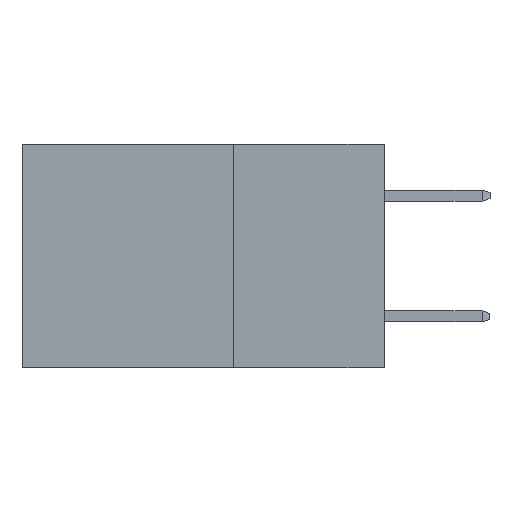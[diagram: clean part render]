
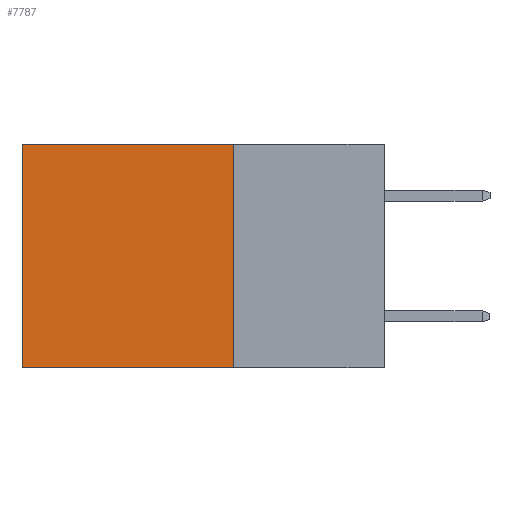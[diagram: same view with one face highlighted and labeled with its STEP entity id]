
A CAD part, left-side view. The second image highlights one B-rep face of the part: STEP entity #7787.
In plain terms, the highlighted planar face has unit normal (-1, 0, 0).
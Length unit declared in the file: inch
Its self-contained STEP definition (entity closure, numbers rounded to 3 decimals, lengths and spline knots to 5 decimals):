
#214 = AXIS2_PLACEMENT_3D ( 'NONE', #4296, #17060, #8611 ) ;
#1659 = LINE ( 'NONE', #11993, #5017 ) ;
#1686 = VERTEX_POINT ( 'NONE', #16379 ) ;
#1791 = CARTESIAN_POINT ( 'NONE',  ( 0.298, 0.6, 0. ) ) ;
#2980 = CARTESIAN_POINT ( 'NONE',  ( 0.298, 0.25, 0. ) ) ;
#3891 = VERTEX_POINT ( 'NONE', #1791 ) ;
#4040 = EDGE_CURVE ( 'NONE', #16604, #3891, #4659, .T. ) ;
#4296 = CARTESIAN_POINT ( 'NONE',  ( 0.298, 0.25, 0. ) ) ;
#4659 = LINE ( 'NONE', #2980, #15600 ) ;
#4667 = DIRECTION ( 'NONE',  ( 0., 1., 0. ) ) ;
#5017 = VECTOR ( 'NONE', #12271, 39.37008 ) ;
#5108 = LINE ( 'NONE', #11768, #16018 ) ;
#6011 = DIRECTION ( 'NONE',  ( 0., 1., 0. ) ) ;
#6279 = EDGE_CURVE ( 'NONE', #16604, #1686, #1659, .T. ) ;
#7108 = CARTESIAN_POINT ( 'NONE',  ( 0.298, 0.6, -0.37 ) ) ;
#7216 = FACE_OUTER_BOUND ( 'NONE', #8972, .T. ) ;
#7787 = ADVANCED_FACE ( 'NONE', ( #7216 ), #8556, .F. ) ;
#8025 = VECTOR ( 'NONE', #14995, 39.37008 ) ;
#8301 = ORIENTED_EDGE ( 'NONE', *, *, #18335, .F. ) ;
#8480 = LINE ( 'NONE', #16353, #8025 ) ;
#8556 = PLANE ( 'NONE',  #214 ) ;
#8611 = DIRECTION ( 'NONE',  ( 0., 0., -1. ) ) ;
#8972 = EDGE_LOOP ( 'NONE', ( #10020, #8301, #13234, #10980 ) ) ;
#9854 = VERTEX_POINT ( 'NONE', #7108 ) ;
#10020 = ORIENTED_EDGE ( 'NONE', *, *, #11534, .T. ) ;
#10980 = ORIENTED_EDGE ( 'NONE', *, *, #4040, .T. ) ;
#11534 = EDGE_CURVE ( 'NONE', #3891, #9854, #8480, .T. ) ;
#11768 = CARTESIAN_POINT ( 'NONE',  ( 0.298, 0.25, -0.37 ) ) ;
#11993 = CARTESIAN_POINT ( 'NONE',  ( 0.298, 0.25, 0. ) ) ;
#12271 = DIRECTION ( 'NONE',  ( 0., 0., -1. ) ) ;
#13234 = ORIENTED_EDGE ( 'NONE', *, *, #6279, .F. ) ;
#14995 = DIRECTION ( 'NONE',  ( 0., 0., -1. ) ) ;
#15600 = VECTOR ( 'NONE', #4667, 39.37008 ) ;
#16018 = VECTOR ( 'NONE', #6011, 39.37008 ) ;
#16353 = CARTESIAN_POINT ( 'NONE',  ( 0.298, 0.6, 0. ) ) ;
#16379 = CARTESIAN_POINT ( 'NONE',  ( 0.298, 0.25, -0.37 ) ) ;
#16604 = VERTEX_POINT ( 'NONE', #17763 ) ;
#17060 = DIRECTION ( 'NONE',  ( 1., 0., 0. ) ) ;
#17763 = CARTESIAN_POINT ( 'NONE',  ( 0.298, 0.25, 0. ) ) ;
#18335 = EDGE_CURVE ( 'NONE', #1686, #9854, #5108, .T. ) ;
